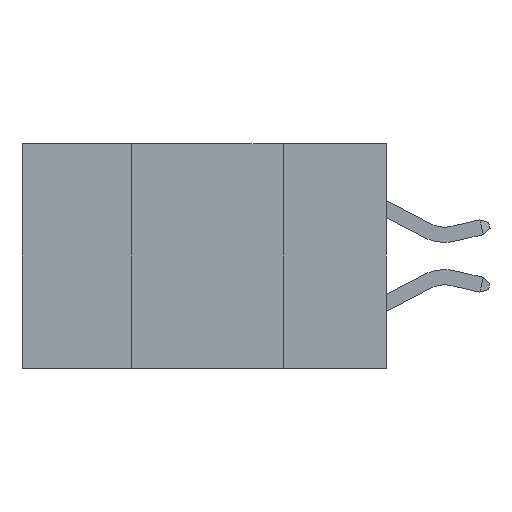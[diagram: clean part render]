
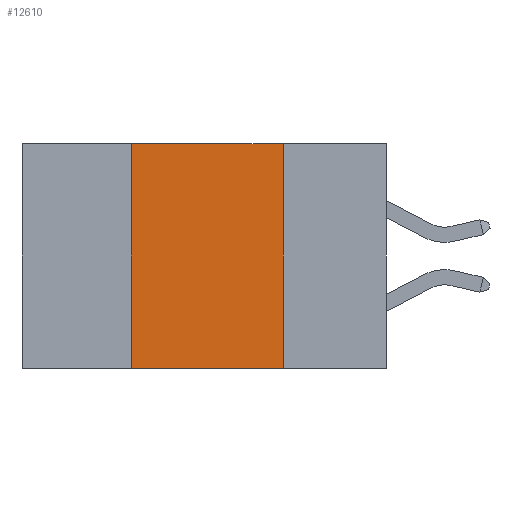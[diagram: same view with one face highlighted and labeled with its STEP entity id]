
A CAD part, left-side view. The second image highlights one B-rep face of the part: STEP entity #12610.
In plain terms, the highlighted planar face has unit normal (-1, 0, 0).
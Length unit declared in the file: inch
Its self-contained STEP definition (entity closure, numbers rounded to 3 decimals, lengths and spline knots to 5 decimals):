
#728 = DIRECTION ( 'NONE',  ( 1., 0., 0. ) ) ;
#1607 = CARTESIAN_POINT ( 'NONE',  ( 0., 0.42, 0. ) ) ;
#1963 = EDGE_LOOP ( 'NONE', ( #16439, #21028, #21618, #22200 ) ) ;
#2542 = PLANE ( 'NONE',  #6813 ) ;
#2928 = VECTOR ( 'NONE', #6370, 39.37008 ) ;
#3973 = LINE ( 'NONE', #11627, #18478 ) ;
#4459 = CARTESIAN_POINT ( 'NONE',  ( 0., 0.17, 0. ) ) ;
#4831 = VECTOR ( 'NONE', #22084, 39.37008 ) ;
#4966 = EDGE_CURVE ( 'NONE', #14251, #23824, #19876, .T. ) ;
#5190 = CARTESIAN_POINT ( 'NONE',  ( 0., 0.17, 0. ) ) ;
#6055 = CARTESIAN_POINT ( 'NONE',  ( 0., 0.17, -0.37 ) ) ;
#6370 = DIRECTION ( 'NONE',  ( 0., 0., 1. ) ) ;
#6813 = AXIS2_PLACEMENT_3D ( 'NONE', #21481, #728, #14084 ) ;
#8001 = LINE ( 'NONE', #19456, #2928 ) ;
#10068 = FACE_OUTER_BOUND ( 'NONE', #1963, .T. ) ;
#10292 = VECTOR ( 'NONE', #17267, 39.37008 ) ;
#10391 = VERTEX_POINT ( 'NONE', #1607 ) ;
#11353 = EDGE_CURVE ( 'NONE', #23460, #10391, #8001, .T. ) ;
#11627 = CARTESIAN_POINT ( 'NONE',  ( 0., 0.6, 0. ) ) ;
#12610 = ADVANCED_FACE ( 'NONE', ( #10068 ), #2542, .F. ) ;
#14084 = DIRECTION ( 'NONE',  ( 0., 0., -1. ) ) ;
#14251 = VERTEX_POINT ( 'NONE', #4459 ) ;
#15371 = CARTESIAN_POINT ( 'NONE',  ( 0., 0.6, -0.37 ) ) ;
#15428 = DIRECTION ( 'NONE',  ( 0., -1., 0. ) ) ;
#15895 = LINE ( 'NONE', #15371, #10292 ) ;
#16437 = CARTESIAN_POINT ( 'NONE',  ( 0., 0.42, -0.37 ) ) ;
#16439 = ORIENTED_EDGE ( 'NONE', *, *, #4966, .F. ) ;
#16703 = EDGE_CURVE ( 'NONE', #10391, #14251, #3973, .T. ) ;
#17267 = DIRECTION ( 'NONE',  ( 0., -1., 0. ) ) ;
#18478 = VECTOR ( 'NONE', #15428, 39.37008 ) ;
#19456 = CARTESIAN_POINT ( 'NONE',  ( 0., 0.42, 0. ) ) ;
#19876 = LINE ( 'NONE', #5190, #4831 ) ;
#21028 = ORIENTED_EDGE ( 'NONE', *, *, #16703, .F. ) ;
#21326 = EDGE_CURVE ( 'NONE', #23460, #23824, #15895, .T. ) ;
#21481 = CARTESIAN_POINT ( 'NONE',  ( 0., 0.6, 0. ) ) ;
#21618 = ORIENTED_EDGE ( 'NONE', *, *, #11353, .F. ) ;
#22084 = DIRECTION ( 'NONE',  ( 0., 0., -1. ) ) ;
#22200 = ORIENTED_EDGE ( 'NONE', *, *, #21326, .T. ) ;
#23460 = VERTEX_POINT ( 'NONE', #16437 ) ;
#23824 = VERTEX_POINT ( 'NONE', #6055 ) ;
